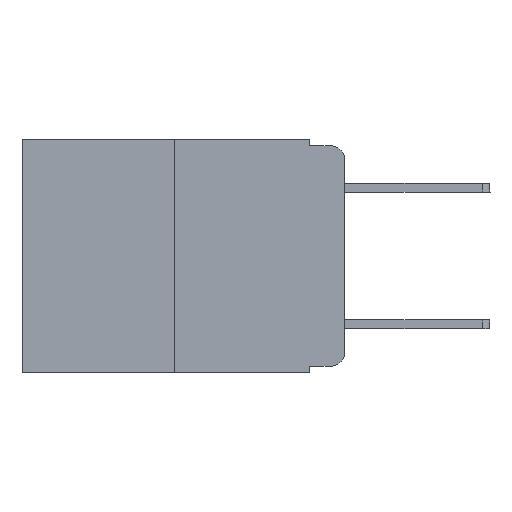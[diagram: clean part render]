
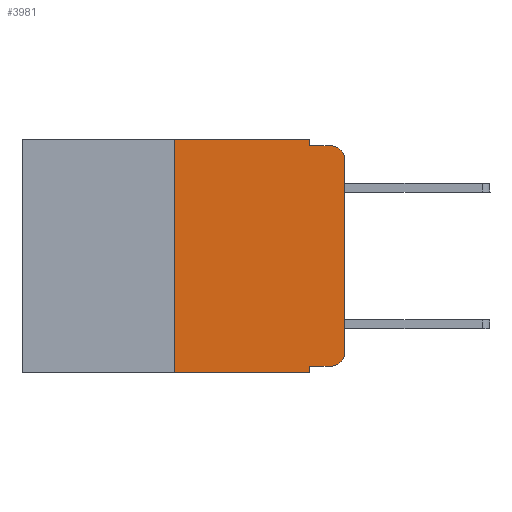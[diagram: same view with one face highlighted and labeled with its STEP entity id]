
A CAD part, left-side view. The second image highlights one B-rep face of the part: STEP entity #3981.
In plain terms, the highlighted planar face has unit normal (-1, 0, 0).
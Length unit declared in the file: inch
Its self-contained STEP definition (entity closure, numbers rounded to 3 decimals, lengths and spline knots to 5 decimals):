
#194 = DIRECTION ( 'NONE',  ( 0., -1., 0. ) ) ;
#984 = VECTOR ( 'NONE', #5729, 39.37008 ) ;
#1086 = AXIS2_PLACEMENT_3D ( 'NONE', #11381, #15857, #3684 ) ;
#1320 = CARTESIAN_POINT ( 'NONE',  ( 0., 0.051, -0.01 ) ) ;
#1441 = EDGE_CURVE ( 'NONE', #14244, #9156, #14709, .T. ) ;
#1466 = ORIENTED_EDGE ( 'NONE', *, *, #5979, .F. ) ;
#1985 = VECTOR ( 'NONE', #4917, 39.37008 ) ;
#2141 = CARTESIAN_POINT ( 'NONE',  ( 0., 0.051, -0.333 ) ) ;
#2628 = DIRECTION ( 'NONE',  ( 0., -1., 0. ) ) ;
#2930 = VERTEX_POINT ( 'NONE', #1320 ) ;
#3230 = CARTESIAN_POINT ( 'NONE',  ( 0., 0., 0. ) ) ;
#3539 = LINE ( 'NONE', #12447, #6263 ) ;
#3664 = VECTOR ( 'NONE', #13032, 39.37008 ) ;
#3684 = DIRECTION ( 'NONE',  ( 0., 0., -1. ) ) ;
#3723 = VERTEX_POINT ( 'NONE', #13405 ) ;
#3920 = DIRECTION ( 'NONE',  ( 0., 0., -1. ) ) ;
#3981 = ADVANCED_FACE ( 'NONE', ( #11581 ), #19340, .F. ) ;
#4392 = EDGE_CURVE ( 'NONE', #3723, #8019, #8538, .T. ) ;
#4917 = DIRECTION ( 'NONE',  ( 0., -1., 0. ) ) ;
#4925 = LINE ( 'NONE', #3230, #17520 ) ;
#4976 = VERTEX_POINT ( 'NONE', #13692 ) ;
#5164 = ORIENTED_EDGE ( 'NONE', *, *, #13485, .T. ) ;
#5376 = ORIENTED_EDGE ( 'NONE', *, *, #17114, .T. ) ;
#5493 = CARTESIAN_POINT ( 'NONE',  ( 0., 0.051, -0.343 ) ) ;
#5729 = DIRECTION ( 'NONE',  ( 0., 0., 1. ) ) ;
#5979 = EDGE_CURVE ( 'NONE', #10619, #8019, #3539, .T. ) ;
#6183 = LINE ( 'NONE', #12284, #13662 ) ;
#6263 = VECTOR ( 'NONE', #18705, 39.37008 ) ;
#6309 = CIRCLE ( 'NONE', #11110, 0.02 ) ;
#6534 = CARTESIAN_POINT ( 'NONE',  ( 0., 0.051, 0. ) ) ;
#6630 = CARTESIAN_POINT ( 'NONE',  ( 0., 0., -0.313 ) ) ;
#6747 = VECTOR ( 'NONE', #3920, 39.37008 ) ;
#6775 = ORIENTED_EDGE ( 'NONE', *, *, #18171, .F. ) ;
#6797 = CARTESIAN_POINT ( 'NONE',  ( 0., 0.25, 0. ) ) ;
#6848 = ORIENTED_EDGE ( 'NONE', *, *, #18648, .F. ) ;
#6870 = DIRECTION ( 'NONE',  ( -1., 0., 0. ) ) ;
#6920 = LINE ( 'NONE', #13022, #6747 ) ;
#7126 = CARTESIAN_POINT ( 'NONE',  ( 0., 0.473, 0. ) ) ;
#7280 = EDGE_LOOP ( 'NONE', ( #5376, #5164, #17435, #6848, #15201, #6775, #15346, #1466, #15660, #11669 ) ) ;
#7788 = EDGE_CURVE ( 'NONE', #2930, #11677, #11215, .T. ) ;
#8019 = VERTEX_POINT ( 'NONE', #5493 ) ;
#8032 = DIRECTION ( 'NONE',  ( 0., 0., 1. ) ) ;
#8538 = LINE ( 'NONE', #19196, #3664 ) ;
#8645 = AXIS2_PLACEMENT_3D ( 'NONE', #12774, #6870, #11374 ) ;
#8749 = CARTESIAN_POINT ( 'NONE',  ( 0., 0.25, 0. ) ) ;
#9156 = VERTEX_POINT ( 'NONE', #6534 ) ;
#9273 = CIRCLE ( 'NONE', #8645, 0.02 ) ;
#10359 = DIRECTION ( 'NONE',  ( 0., 0., -1. ) ) ;
#10570 = VERTEX_POINT ( 'NONE', #6630 ) ;
#10619 = VERTEX_POINT ( 'NONE', #2141 ) ;
#10797 = CARTESIAN_POINT ( 'NONE',  ( 0., 0., -0.03 ) ) ;
#11110 = AXIS2_PLACEMENT_3D ( 'NONE', #13448, #13542, #10359 ) ;
#11215 = LINE ( 'NONE', #18585, #1985 ) ;
#11374 = DIRECTION ( 'NONE',  ( 0., 0., -1. ) ) ;
#11381 = CARTESIAN_POINT ( 'NONE',  ( 0., 0.473, 0. ) ) ;
#11581 = FACE_OUTER_BOUND ( 'NONE', #7280, .T. ) ;
#11669 = ORIENTED_EDGE ( 'NONE', *, *, #17606, .T. ) ;
#11677 = VERTEX_POINT ( 'NONE', #15937 ) ;
#12284 = CARTESIAN_POINT ( 'NONE',  ( 0., 0.051, -0.333 ) ) ;
#12447 = CARTESIAN_POINT ( 'NONE',  ( 0., 0.051, 0. ) ) ;
#12774 = CARTESIAN_POINT ( 'NONE',  ( 0., 0.02, -0.313 ) ) ;
#13022 = CARTESIAN_POINT ( 'NONE',  ( 0., 0.051, 0. ) ) ;
#13032 = DIRECTION ( 'NONE',  ( 0., -1., 0. ) ) ;
#13241 = EDGE_CURVE ( 'NONE', #10619, #4976, #6183, .T. ) ;
#13405 = CARTESIAN_POINT ( 'NONE',  ( 0., 0.25, -0.343 ) ) ;
#13448 = CARTESIAN_POINT ( 'NONE',  ( 0., 0.02, -0.03 ) ) ;
#13485 = EDGE_CURVE ( 'NONE', #19388, #11677, #6309, .T. ) ;
#13542 = DIRECTION ( 'NONE',  ( -1., 0., 0. ) ) ;
#13662 = VECTOR ( 'NONE', #194, 39.37008 ) ;
#13692 = CARTESIAN_POINT ( 'NONE',  ( 0., 0.02, -0.333 ) ) ;
#14244 = VERTEX_POINT ( 'NONE', #6797 ) ;
#14709 = LINE ( 'NONE', #7126, #18858 ) ;
#15201 = ORIENTED_EDGE ( 'NONE', *, *, #1441, .F. ) ;
#15346 = ORIENTED_EDGE ( 'NONE', *, *, #4392, .T. ) ;
#15660 = ORIENTED_EDGE ( 'NONE', *, *, #13241, .T. ) ;
#15857 = DIRECTION ( 'NONE',  ( 1., 0., 0. ) ) ;
#15937 = CARTESIAN_POINT ( 'NONE',  ( 0., 0.02, -0.01 ) ) ;
#16214 = LINE ( 'NONE', #8749, #984 ) ;
#17114 = EDGE_CURVE ( 'NONE', #10570, #19388, #4925, .T. ) ;
#17435 = ORIENTED_EDGE ( 'NONE', *, *, #7788, .F. ) ;
#17520 = VECTOR ( 'NONE', #8032, 39.37008 ) ;
#17606 = EDGE_CURVE ( 'NONE', #4976, #10570, #9273, .T. ) ;
#18171 = EDGE_CURVE ( 'NONE', #3723, #14244, #16214, .T. ) ;
#18585 = CARTESIAN_POINT ( 'NONE',  ( 0., 0.051, -0.01 ) ) ;
#18648 = EDGE_CURVE ( 'NONE', #9156, #2930, #6920, .T. ) ;
#18705 = DIRECTION ( 'NONE',  ( 0., 0., -1. ) ) ;
#18858 = VECTOR ( 'NONE', #2628, 39.37008 ) ;
#19196 = CARTESIAN_POINT ( 'NONE',  ( 0., 0.473, -0.343 ) ) ;
#19340 = PLANE ( 'NONE',  #1086 ) ;
#19388 = VERTEX_POINT ( 'NONE', #10797 ) ;
